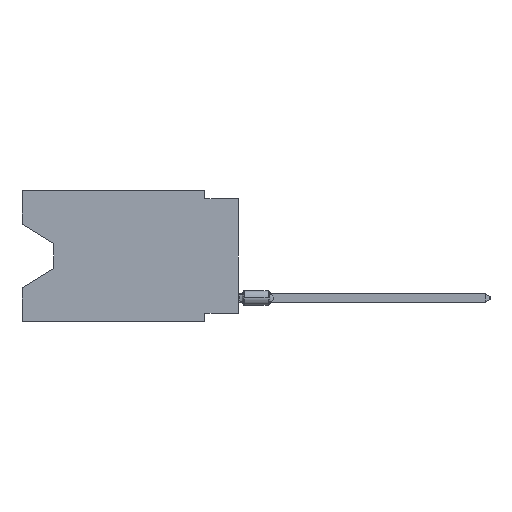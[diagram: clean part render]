
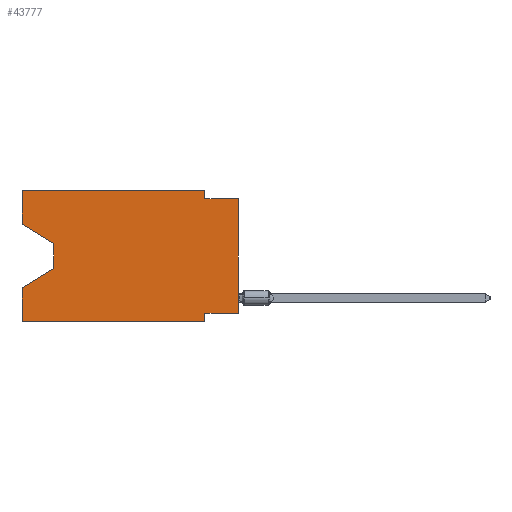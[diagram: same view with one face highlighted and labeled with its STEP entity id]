
A CAD part, left-side view. The second image highlights one B-rep face of the part: STEP entity #43777.
In plain terms, the highlighted planar face has unit normal (-1, 0, 0).
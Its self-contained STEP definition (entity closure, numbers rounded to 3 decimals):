
#90 = CARTESIAN_POINT ( 'NONE',  ( 0., 2.54, -9.906 ) ) ;
#495 = EDGE_CURVE ( 'NONE', #37105, #1760, #36006, .T. ) ;
#507 = VECTOR ( 'NONE', #44641, 1000. ) ;
#659 = ORIENTED_EDGE ( 'NONE', *, *, #38288, .F. ) ;
#799 = CARTESIAN_POINT ( 'NONE',  ( 0., 16.383, -2.546 ) ) ;
#1760 = VERTEX_POINT ( 'NONE', #17130 ) ;
#2585 = VECTOR ( 'NONE', #45036, 1000. ) ;
#2626 = CARTESIAN_POINT ( 'NONE',  ( 0., 2.54, -9.906 ) ) ;
#4412 = CARTESIAN_POINT ( 'NONE',  ( 0., 2.54, -0.635 ) ) ;
#4646 = ORIENTED_EDGE ( 'NONE', *, *, #20045, .T. ) ;
#4858 = VERTEX_POINT ( 'NONE', #40456 ) ;
#5990 = DIRECTION ( 'NONE',  ( 1., 0., 0. ) ) ;
#6176 = ORIENTED_EDGE ( 'NONE', *, *, #16172, .F. ) ;
#7226 = LINE ( 'NONE', #37736, #52311 ) ;
#7791 = DIRECTION ( 'NONE',  ( 0., 0., -1. ) ) ;
#7912 = EDGE_CURVE ( 'NONE', #51081, #54170, #28009, .T. ) ;
#9452 = DIRECTION ( 'NONE',  ( 0., 0., 1. ) ) ;
#9602 = LINE ( 'NONE', #52375, #53522 ) ;
#9668 = VECTOR ( 'NONE', #18291, 1000. ) ;
#9695 = CARTESIAN_POINT ( 'NONE',  ( 0., 13.97, -5.893 ) ) ;
#9709 = VECTOR ( 'NONE', #40181, 1000. ) ;
#11017 = ORIENTED_EDGE ( 'NONE', *, *, #46436, .F. ) ;
#12432 = CARTESIAN_POINT ( 'NONE',  ( 0., 16.383, -2.546 ) ) ;
#13217 = LINE ( 'NONE', #90, #22387 ) ;
#13230 = CARTESIAN_POINT ( 'NONE',  ( 0., 13.97, -4.013 ) ) ;
#13798 = EDGE_LOOP ( 'NONE', ( #4646, #46135, #19836, #49872, #46672, #27511, #6176, #24660, #45786, #11017, #43603, #659 ) ) ;
#14329 = VERTEX_POINT ( 'NONE', #12432 ) ;
#16056 = DIRECTION ( 'NONE',  ( 0., 0., 1. ) ) ;
#16172 = EDGE_CURVE ( 'NONE', #38345, #26484, #9602, .T. ) ;
#17130 = CARTESIAN_POINT ( 'NONE',  ( 0., 16.383, -7.36 ) ) ;
#18291 = DIRECTION ( 'NONE',  ( 0., -1., 0. ) ) ;
#18387 = CARTESIAN_POINT ( 'NONE',  ( 0., 13.97, -4.013 ) ) ;
#18558 = LINE ( 'NONE', #53182, #9668 ) ;
#18668 = LINE ( 'NONE', #22314, #507 ) ;
#18709 = LINE ( 'NONE', #35766, #39041 ) ;
#19178 = DIRECTION ( 'NONE',  ( 0., 0., -1. ) ) ;
#19836 = ORIENTED_EDGE ( 'NONE', *, *, #495, .T. ) ;
#20045 = EDGE_CURVE ( 'NONE', #14329, #43995, #22074, .T. ) ;
#20099 = VERTEX_POINT ( 'NONE', #4412 ) ;
#22074 = LINE ( 'NONE', #799, #47791 ) ;
#22314 = CARTESIAN_POINT ( 'NONE',  ( 0., 16.383, 0. ) ) ;
#22387 = VECTOR ( 'NONE', #30570, 1000. ) ;
#24623 = CARTESIAN_POINT ( 'NONE',  ( 0., 2.54, 0. ) ) ;
#24660 = ORIENTED_EDGE ( 'NONE', *, *, #40659, .T. ) ;
#26184 = VECTOR ( 'NONE', #39070, 1000. ) ;
#26484 = VERTEX_POINT ( 'NONE', #47398 ) ;
#27005 = FACE_OUTER_BOUND ( 'NONE', #13798, .T. ) ;
#27463 = EDGE_CURVE ( 'NONE', #51081, #1760, #7226, .T. ) ;
#27511 = ORIENTED_EDGE ( 'NONE', *, *, #38475, .F. ) ;
#28009 = LINE ( 'NONE', #48934, #2585 ) ;
#30570 = DIRECTION ( 'NONE',  ( 0., 0., -1. ) ) ;
#32889 = EDGE_CURVE ( 'NONE', #41486, #37488, #18668, .T. ) ;
#35163 = AXIS2_PLACEMENT_3D ( 'NONE', #40416, #5990, #19178 ) ;
#35766 = CARTESIAN_POINT ( 'NONE',  ( 0., 0., 0. ) ) ;
#35917 = DIRECTION ( 'NONE',  ( 0., 1., 0. ) ) ;
#36006 = LINE ( 'NONE', #9695, #9709 ) ;
#37105 = VERTEX_POINT ( 'NONE', #37184 ) ;
#37184 = CARTESIAN_POINT ( 'NONE',  ( 0., 13.97, -5.893 ) ) ;
#37325 = LINE ( 'NONE', #55145, #44657 ) ;
#37475 = LINE ( 'NONE', #24623, #38427 ) ;
#37488 = VERTEX_POINT ( 'NONE', #37868 ) ;
#37736 = CARTESIAN_POINT ( 'NONE',  ( 0., 16.383, 0. ) ) ;
#37868 = CARTESIAN_POINT ( 'NONE',  ( 0., 2.54, 0. ) ) ;
#38288 = EDGE_CURVE ( 'NONE', #14329, #41486, #37325, .T. ) ;
#38345 = VERTEX_POINT ( 'NONE', #49856 ) ;
#38427 = VECTOR ( 'NONE', #7791, 1000. ) ;
#38475 = EDGE_CURVE ( 'NONE', #26484, #54170, #13217, .T. ) ;
#39041 = VECTOR ( 'NONE', #9452, 1000. ) ;
#39070 = DIRECTION ( 'NONE',  ( 0., 0., -1. ) ) ;
#40181 = DIRECTION ( 'NONE',  ( 0., 0.855, -0.519 ) ) ;
#40416 = CARTESIAN_POINT ( 'NONE',  ( 0., 16.383, 0. ) ) ;
#40456 = CARTESIAN_POINT ( 'NONE',  ( 0., 0., -0.635 ) ) ;
#40659 = EDGE_CURVE ( 'NONE', #38345, #4858, #18709, .T. ) ;
#41486 = VERTEX_POINT ( 'NONE', #53957 ) ;
#43603 = ORIENTED_EDGE ( 'NONE', *, *, #32889, .F. ) ;
#43777 = ADVANCED_FACE ( 'NONE', ( #27005 ), #52137, .F. ) ;
#43995 = VERTEX_POINT ( 'NONE', #13230 ) ;
#44085 = LINE ( 'NONE', #18387, #26184 ) ;
#44641 = DIRECTION ( 'NONE',  ( 0., -1., 0. ) ) ;
#44657 = VECTOR ( 'NONE', #16056, 1000. ) ;
#45036 = DIRECTION ( 'NONE',  ( 0., -1., 0. ) ) ;
#45418 = EDGE_CURVE ( 'NONE', #20099, #4858, #18558, .T. ) ;
#45786 = ORIENTED_EDGE ( 'NONE', *, *, #45418, .F. ) ;
#46085 = DIRECTION ( 'NONE',  ( 0., 0., 1. ) ) ;
#46135 = ORIENTED_EDGE ( 'NONE', *, *, #50346, .T. ) ;
#46436 = EDGE_CURVE ( 'NONE', #37488, #20099, #37475, .T. ) ;
#46672 = ORIENTED_EDGE ( 'NONE', *, *, #7912, .T. ) ;
#47398 = CARTESIAN_POINT ( 'NONE',  ( 0., 2.54, -9.271 ) ) ;
#47791 = VECTOR ( 'NONE', #50839, 1000. ) ;
#48934 = CARTESIAN_POINT ( 'NONE',  ( 0., 16.383, -9.906 ) ) ;
#49856 = CARTESIAN_POINT ( 'NONE',  ( 0., 0., -9.271 ) ) ;
#49872 = ORIENTED_EDGE ( 'NONE', *, *, #27463, .F. ) ;
#50346 = EDGE_CURVE ( 'NONE', #43995, #37105, #44085, .T. ) ;
#50839 = DIRECTION ( 'NONE',  ( 0., -0.855, -0.519 ) ) ;
#51081 = VERTEX_POINT ( 'NONE', #54325 ) ;
#52137 = PLANE ( 'NONE',  #35163 ) ;
#52311 = VECTOR ( 'NONE', #46085, 1000. ) ;
#52375 = CARTESIAN_POINT ( 'NONE',  ( 0., 0., -9.271 ) ) ;
#53182 = CARTESIAN_POINT ( 'NONE',  ( 0., 0., -0.635 ) ) ;
#53522 = VECTOR ( 'NONE', #35917, 1000. ) ;
#53957 = CARTESIAN_POINT ( 'NONE',  ( 0., 16.383, 0. ) ) ;
#54170 = VERTEX_POINT ( 'NONE', #2626 ) ;
#54325 = CARTESIAN_POINT ( 'NONE',  ( 0., 16.383, -9.906 ) ) ;
#55145 = CARTESIAN_POINT ( 'NONE',  ( 0., 16.383, 0. ) ) ;
